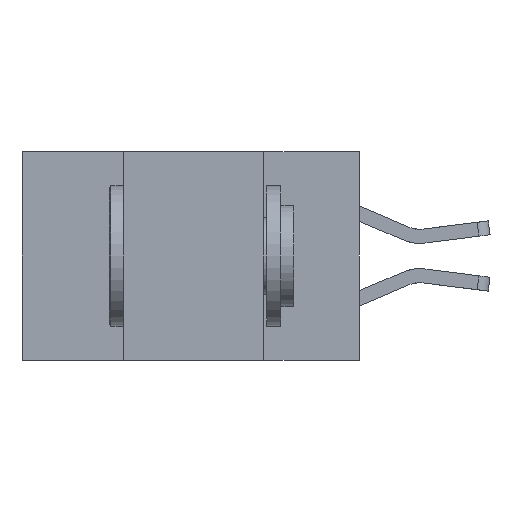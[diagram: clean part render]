
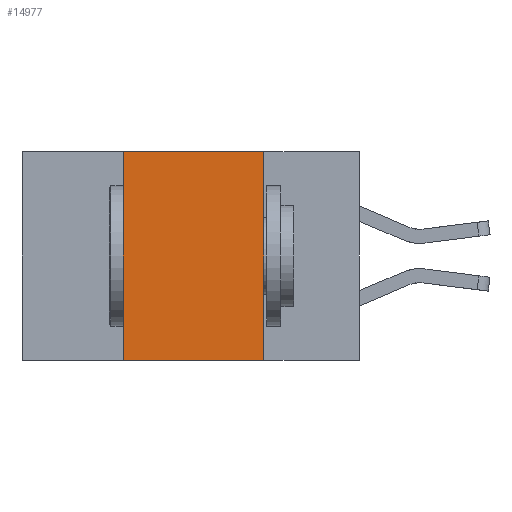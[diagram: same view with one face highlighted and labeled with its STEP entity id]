
A CAD part, left-side view. The second image highlights one B-rep face of the part: STEP entity #14977.
In plain terms, the highlighted planar face has unit normal (-1, 0, 0).
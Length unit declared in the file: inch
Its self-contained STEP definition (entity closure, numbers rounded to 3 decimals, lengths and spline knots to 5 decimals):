
#21 = DIRECTION ( 'NONE',  ( 1., 0., 0. ) ) ;
#743 = FACE_OUTER_BOUND ( 'NONE', #5801, .T. ) ;
#892 = VECTOR ( 'NONE', #12195, 39.37008 ) ;
#2361 = VECTOR ( 'NONE', #10802, 39.37008 ) ;
#2901 = LINE ( 'NONE', #8031, #12362 ) ;
#3030 = CARTESIAN_POINT ( 'NONE',  ( 0., 0.42, 0. ) ) ;
#3192 = EDGE_CURVE ( 'NONE', #10519, #9915, #12554, .T. ) ;
#3264 = DIRECTION ( 'NONE',  ( 0., 0., 1. ) ) ;
#3706 = LINE ( 'NONE', #11913, #15864 ) ;
#4974 = CARTESIAN_POINT ( 'NONE',  ( 0., 0.6, 0. ) ) ;
#5445 = VERTEX_POINT ( 'NONE', #9606 ) ;
#5510 = EDGE_CURVE ( 'NONE', #9915, #7296, #13957, .T. ) ;
#5801 = EDGE_LOOP ( 'NONE', ( #15697, #15737, #15851, #13936 ) ) ;
#6426 = AXIS2_PLACEMENT_3D ( 'NONE', #4974, #21, #8709 ) ;
#7296 = VERTEX_POINT ( 'NONE', #8200 ) ;
#8031 = CARTESIAN_POINT ( 'NONE',  ( 0., 0.6, -0.37 ) ) ;
#8200 = CARTESIAN_POINT ( 'NONE',  ( 0., 0.17, -0.37 ) ) ;
#8709 = DIRECTION ( 'NONE',  ( 0., 0., -1. ) ) ;
#8921 = CARTESIAN_POINT ( 'NONE',  ( 0., 0.6, 0. ) ) ;
#9326 = DIRECTION ( 'NONE',  ( 0., -1., 0. ) ) ;
#9406 = EDGE_CURVE ( 'NONE', #5445, #10519, #3706, .T. ) ;
#9606 = CARTESIAN_POINT ( 'NONE',  ( 0., 0.42, -0.37 ) ) ;
#9915 = VERTEX_POINT ( 'NONE', #15117 ) ;
#10519 = VERTEX_POINT ( 'NONE', #3030 ) ;
#10802 = DIRECTION ( 'NONE',  ( 0., -1., 0. ) ) ;
#11113 = EDGE_CURVE ( 'NONE', #5445, #7296, #2901, .T. ) ;
#11913 = CARTESIAN_POINT ( 'NONE',  ( 0., 0.42, 0. ) ) ;
#12195 = DIRECTION ( 'NONE',  ( 0., 0., -1. ) ) ;
#12362 = VECTOR ( 'NONE', #9326, 39.37008 ) ;
#12406 = PLANE ( 'NONE',  #6426 ) ;
#12554 = LINE ( 'NONE', #8921, #2361 ) ;
#13936 = ORIENTED_EDGE ( 'NONE', *, *, #11113, .T. ) ;
#13957 = LINE ( 'NONE', #14487, #892 ) ;
#14487 = CARTESIAN_POINT ( 'NONE',  ( 0., 0.17, 0. ) ) ;
#14977 = ADVANCED_FACE ( 'NONE', ( #743 ), #12406, .F. ) ;
#15117 = CARTESIAN_POINT ( 'NONE',  ( 0., 0.17, 0. ) ) ;
#15697 = ORIENTED_EDGE ( 'NONE', *, *, #5510, .F. ) ;
#15737 = ORIENTED_EDGE ( 'NONE', *, *, #3192, .F. ) ;
#15851 = ORIENTED_EDGE ( 'NONE', *, *, #9406, .F. ) ;
#15864 = VECTOR ( 'NONE', #3264, 39.37008 ) ;
